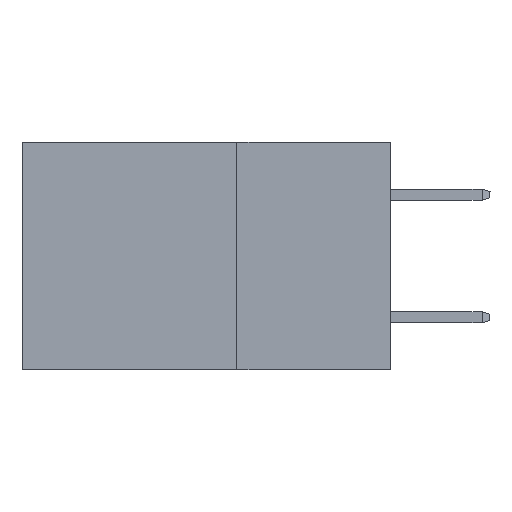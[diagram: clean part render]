
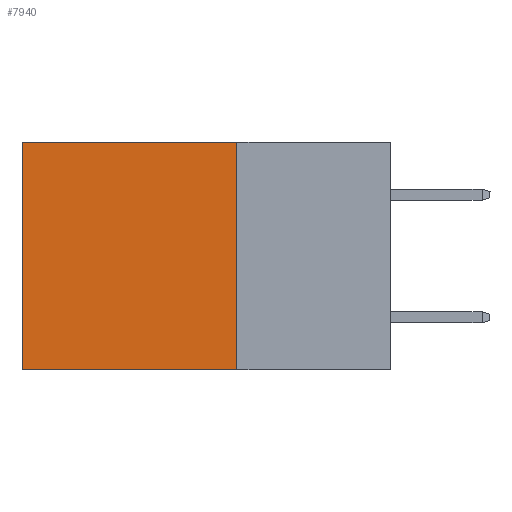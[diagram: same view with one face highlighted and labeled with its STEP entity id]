
A CAD part, left-side view. The second image highlights one B-rep face of the part: STEP entity #7940.
In plain terms, the highlighted planar face has unit normal (-1, 0, 0).
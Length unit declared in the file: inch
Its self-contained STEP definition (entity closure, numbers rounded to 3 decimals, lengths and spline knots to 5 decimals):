
#1526 = CARTESIAN_POINT ( 'NONE',  ( 0.2875, 0.25, -0.37 ) ) ;
#1954 = CARTESIAN_POINT ( 'NONE',  ( 0.2875, 0.25, -0.37 ) ) ;
#2074 = CARTESIAN_POINT ( 'NONE',  ( 0.2875, 0.25, 0. ) ) ;
#2846 = EDGE_CURVE ( 'NONE', #16407, #14894, #7335, .T. ) ;
#3434 = AXIS2_PLACEMENT_3D ( 'NONE', #18991, #14933, #11068 ) ;
#3647 = ORIENTED_EDGE ( 'NONE', *, *, #5717, .F. ) ;
#3779 = FACE_OUTER_BOUND ( 'NONE', #18243, .T. ) ;
#3788 = CARTESIAN_POINT ( 'NONE',  ( 0.2875, 0.6, 0. ) ) ;
#3863 = ORIENTED_EDGE ( 'NONE', *, *, #10381, .F. ) ;
#3925 = LINE ( 'NONE', #2074, #20358 ) ;
#4781 = CARTESIAN_POINT ( 'NONE',  ( 0.2875, 0.6, 0. ) ) ;
#5024 = CARTESIAN_POINT ( 'NONE',  ( 0.2875, 0.6, -0.37 ) ) ;
#5717 = EDGE_CURVE ( 'NONE', #11498, #8766, #16516, .T. ) ;
#7335 = LINE ( 'NONE', #14036, #15372 ) ;
#7817 = PLANE ( 'NONE',  #3434 ) ;
#7940 = ADVANCED_FACE ( 'NONE', ( #3779 ), #7817, .F. ) ;
#7980 = VECTOR ( 'NONE', #13075, 39.37008 ) ;
#8485 = ORIENTED_EDGE ( 'NONE', *, *, #2846, .T. ) ;
#8766 = VERTEX_POINT ( 'NONE', #5024 ) ;
#9386 = VECTOR ( 'NONE', #17532, 39.37008 ) ;
#10381 = EDGE_CURVE ( 'NONE', #16407, #11498, #3925, .T. ) ;
#10805 = DIRECTION ( 'NONE',  ( 0., 1., 0. ) ) ;
#11068 = DIRECTION ( 'NONE',  ( 0., 0., -1. ) ) ;
#11498 = VERTEX_POINT ( 'NONE', #1526 ) ;
#11607 = DIRECTION ( 'NONE',  ( 0., 0., -1. ) ) ;
#13075 = DIRECTION ( 'NONE',  ( 0., 1., 0. ) ) ;
#14036 = CARTESIAN_POINT ( 'NONE',  ( 0.2875, 0.25, 0. ) ) ;
#14894 = VERTEX_POINT ( 'NONE', #3788 ) ;
#14933 = DIRECTION ( 'NONE',  ( 1., 0., 0. ) ) ;
#15318 = CARTESIAN_POINT ( 'NONE',  ( 0.2875, 0.25, 0. ) ) ;
#15372 = VECTOR ( 'NONE', #10805, 39.37008 ) ;
#15663 = LINE ( 'NONE', #4781, #9386 ) ;
#16407 = VERTEX_POINT ( 'NONE', #15318 ) ;
#16516 = LINE ( 'NONE', #1954, #7980 ) ;
#17532 = DIRECTION ( 'NONE',  ( 0., 0., -1. ) ) ;
#17659 = ORIENTED_EDGE ( 'NONE', *, *, #17850, .T. ) ;
#17850 = EDGE_CURVE ( 'NONE', #14894, #8766, #15663, .T. ) ;
#18243 = EDGE_LOOP ( 'NONE', ( #17659, #3647, #3863, #8485 ) ) ;
#18991 = CARTESIAN_POINT ( 'NONE',  ( 0.2875, 0.25, 0. ) ) ;
#20358 = VECTOR ( 'NONE', #11607, 39.37008 ) ;
